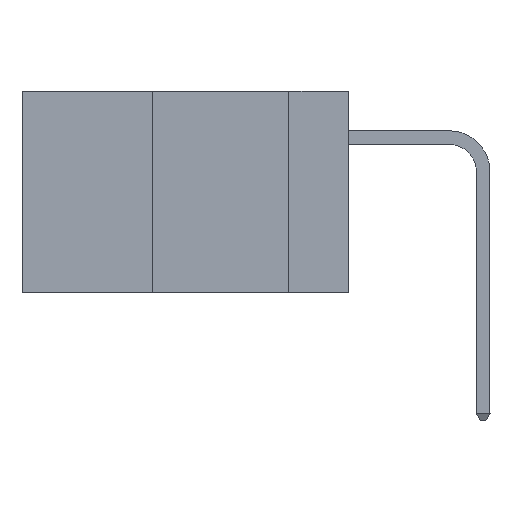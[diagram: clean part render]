
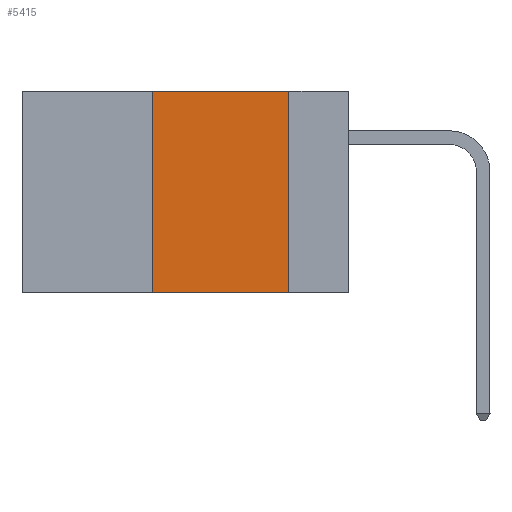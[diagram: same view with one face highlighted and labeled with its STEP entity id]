
A CAD part, left-side view. The second image highlights one B-rep face of the part: STEP entity #5415.
In plain terms, the highlighted planar face has unit normal (-1, 0, 0).
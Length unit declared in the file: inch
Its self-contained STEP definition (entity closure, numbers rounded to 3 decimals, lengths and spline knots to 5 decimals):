
#1951 = DIRECTION ( 'NONE',  ( 0., -1., 0. ) ) ;
#2349 = EDGE_CURVE ( 'NONE', #23909, #41435, #28110, .T. ) ;
#4833 = CARTESIAN_POINT ( 'NONE',  ( 0., 0.36, 0. ) ) ;
#5415 = ADVANCED_FACE ( 'NONE', ( #43223 ), #10072, .F. ) ;
#5667 = CARTESIAN_POINT ( 'NONE',  ( 0., 0.6, -0.37 ) ) ;
#7532 = VERTEX_POINT ( 'NONE', #20732 ) ;
#8341 = DIRECTION ( 'NONE',  ( 0., 0., 1. ) ) ;
#9426 = ORIENTED_EDGE ( 'NONE', *, *, #15571, .F. ) ;
#9587 = DIRECTION ( 'NONE',  ( 0., -1., 0. ) ) ;
#9799 = CARTESIAN_POINT ( 'NONE',  ( 0., 0.6, 0. ) ) ;
#10072 = PLANE ( 'NONE',  #28204 ) ;
#11833 = LINE ( 'NONE', #5667, #18138 ) ;
#11845 = ORIENTED_EDGE ( 'NONE', *, *, #32170, .F. ) ;
#14356 = EDGE_CURVE ( 'NONE', #23909, #7532, #11833, .T. ) ;
#14963 = VERTEX_POINT ( 'NONE', #18806 ) ;
#15571 = EDGE_CURVE ( 'NONE', #14963, #7532, #23339, .T. ) ;
#16956 = DIRECTION ( 'NONE',  ( 0., 0., -1. ) ) ;
#17750 = VECTOR ( 'NONE', #9587, 39.37008 ) ;
#18138 = VECTOR ( 'NONE', #1951, 39.37008 ) ;
#18806 = CARTESIAN_POINT ( 'NONE',  ( 0., 0.11, 0. ) ) ;
#20732 = CARTESIAN_POINT ( 'NONE',  ( 0., 0.11, -0.37 ) ) ;
#22315 = VECTOR ( 'NONE', #16956, 39.37008 ) ;
#23339 = LINE ( 'NONE', #40438, #22315 ) ;
#23479 = CARTESIAN_POINT ( 'NONE',  ( 0., 0.6, 0. ) ) ;
#23909 = VERTEX_POINT ( 'NONE', #34126 ) ;
#28110 = LINE ( 'NONE', #4833, #32211 ) ;
#28204 = AXIS2_PLACEMENT_3D ( 'NONE', #23479, #36198, #36852 ) ;
#31203 = EDGE_LOOP ( 'NONE', ( #9426, #11845, #34699, #36003 ) ) ;
#32170 = EDGE_CURVE ( 'NONE', #41435, #14963, #36142, .T. ) ;
#32211 = VECTOR ( 'NONE', #8341, 39.37008 ) ;
#34126 = CARTESIAN_POINT ( 'NONE',  ( 0., 0.36, -0.37 ) ) ;
#34699 = ORIENTED_EDGE ( 'NONE', *, *, #2349, .F. ) ;
#36003 = ORIENTED_EDGE ( 'NONE', *, *, #14356, .T. ) ;
#36142 = LINE ( 'NONE', #9799, #17750 ) ;
#36198 = DIRECTION ( 'NONE',  ( 1., 0., 0. ) ) ;
#36366 = CARTESIAN_POINT ( 'NONE',  ( 0., 0.36, 0. ) ) ;
#36852 = DIRECTION ( 'NONE',  ( 0., 0., -1. ) ) ;
#40438 = CARTESIAN_POINT ( 'NONE',  ( 0., 0.11, 0. ) ) ;
#41435 = VERTEX_POINT ( 'NONE', #36366 ) ;
#43223 = FACE_OUTER_BOUND ( 'NONE', #31203, .T. ) ;
